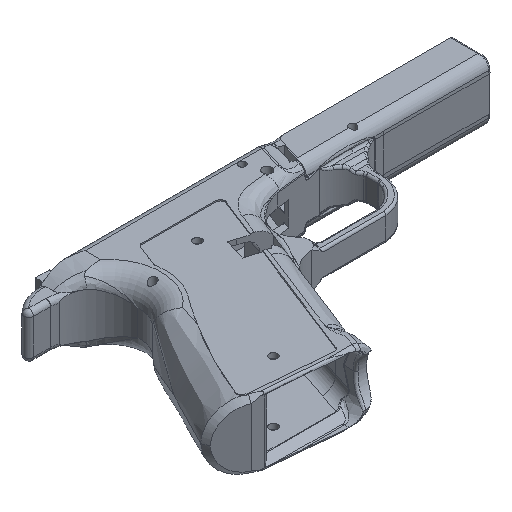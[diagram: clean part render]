
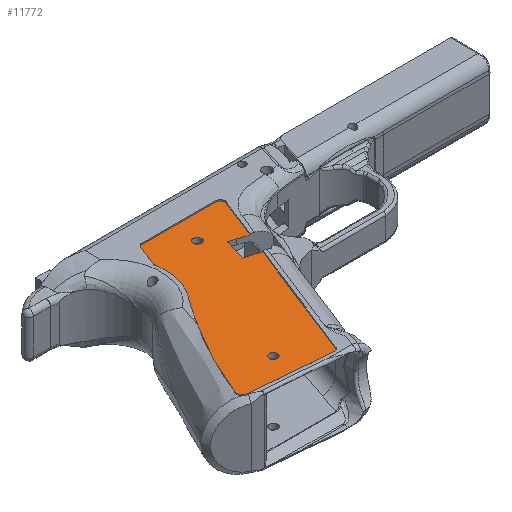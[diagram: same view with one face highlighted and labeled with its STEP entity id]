
A CAD part, isometric view. The second image highlights one B-rep face of the part: STEP entity #11772.
In plain terms, the highlighted planar face has unit normal (0, 0, 1).
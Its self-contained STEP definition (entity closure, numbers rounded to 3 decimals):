
#159=FACE_BOUND('',#2811,.T.);
#160=FACE_BOUND('',#2812,.T.);
#457=B_SPLINE_CURVE_WITH_KNOTS('',3,(#16690,#16691,#16692,#16693),
 .UNSPECIFIED.,.F.,.F.,(4,4),(1.719,2.121),
 .UNSPECIFIED.);
#1124=CIRCLE('',#11847,2.);
#1127=CIRCLE('',#11852,205.915);
#1274=CIRCLE('',#12141,2.);
#1275=CIRCLE('',#12143,22.827);
#1276=CIRCLE('',#12145,2.);
#1277=CIRCLE('',#12149,2.);
#1278=CIRCLE('',#12151,205.915);
#1279=CIRCLE('',#12153,2.);
#1280=CIRCLE('',#12156,2.);
#1281=CIRCLE('',#12162,21.378);
#1524=CIRCLE('',#12781,1.75);
#1526=CIRCLE('',#12784,1.75);
#2159=FACE_OUTER_BOUND('',#2810,.T.);
#2810=EDGE_LOOP('',(#10894,#10895,#10896,#10897,#10898,#10899,#10900,#10901,
#10902,#10903,#10904,#10905,#10906,#10907,#10908,#10909,#10910,#10911,#10912,
#10913));
#2811=EDGE_LOOP('',(#10914));
#2812=EDGE_LOOP('',(#10915));
#3101=LINE('',#24441,#3852);
#3103=LINE('',#24446,#3854);
#3109=LINE('',#24464,#3860);
#3111=LINE('',#24468,#3862);
#3115=LINE('',#24481,#3866);
#3116=LINE('',#24485,#3867);
#3117=LINE('',#24488,#3868);
#3226=LINE('',#29078,#3977);
#3246=LINE('',#29541,#3997);
#3852=VECTOR('',#13776,10.);
#3854=VECTOR('',#13780,10.);
#3860=VECTOR('',#13800,10.);
#3862=VECTOR('',#13804,10.);
#3866=VECTOR('',#13822,10.);
#3867=VECTOR('',#13829,10.);
#3868=VECTOR('',#13832,10.);
#3977=VECTOR('',#14211,10.);
#3997=VECTOR('',#14275,10.);
#4429=VERTEX_POINT('',#16684);
#4430=VERTEX_POINT('',#16689);
#4471=VERTEX_POINT('',#17024);
#4472=VERTEX_POINT('',#17026);
#4479=VERTEX_POINT('',#17115);
#4898=VERTEX_POINT('',#24437);
#4899=VERTEX_POINT('',#24439);
#4900=VERTEX_POINT('',#24443);
#4901=VERTEX_POINT('',#24445);
#4902=VERTEX_POINT('',#24449);
#4903=VERTEX_POINT('',#24450);
#4904=VERTEX_POINT('',#24457);
#4905=VERTEX_POINT('',#24458);
#4906=VERTEX_POINT('',#24463);
#4907=VERTEX_POINT('',#24467);
#4908=VERTEX_POINT('',#24471);
#4909=VERTEX_POINT('',#24477);
#4910=VERTEX_POINT('',#24487);
#4919=VERTEX_POINT('',#24523);
#5103=VERTEX_POINT('',#29077);
#5481=VERTEX_POINT('',#37650);
#5483=VERTEX_POINT('',#37656);
#5615=EDGE_CURVE('',#4429,#4430,#457,.T.);
#5663=EDGE_CURVE('',#4471,#4472,#1124,.T.);
#5672=EDGE_CURVE('',#4479,#4430,#1127,.T.);
#6277=EDGE_CURVE('',#4898,#4899,#3101,.T.);
#6279=EDGE_CURVE('',#4901,#4900,#3103,.T.);
#6281=EDGE_CURVE('',#4902,#4903,#1274,.T.);
#6284=EDGE_CURVE('',#4902,#4479,#1275,.T.);
#6285=EDGE_CURVE('',#4904,#4905,#1276,.T.);
#6288=EDGE_CURVE('',#4906,#4905,#3109,.T.);
#6290=EDGE_CURVE('',#4907,#4472,#3111,.T.);
#6292=EDGE_CURVE('',#4907,#4908,#1277,.T.);
#6294=EDGE_CURVE('',#4429,#4908,#1278,.T.);
#6295=EDGE_CURVE('',#4901,#4909,#1279,.T.);
#6297=EDGE_CURVE('',#4471,#4909,#3115,.T.);
#6298=EDGE_CURVE('',#4906,#4899,#1280,.T.);
#6299=EDGE_CURVE('',#4904,#4903,#3116,.T.);
#6300=EDGE_CURVE('',#4910,#4898,#3117,.T.);
#6310=EDGE_CURVE('',#4919,#4910,#1281,.T.);
#6587=EDGE_CURVE('',#5103,#4919,#3226,.T.);
#6622=EDGE_CURVE('',#4900,#5103,#3246,.T.);
#7296=EDGE_CURVE('',#5481,#5481,#1524,.T.);
#7299=EDGE_CURVE('',#5483,#5483,#1526,.T.);
#10894=ORIENTED_EDGE('',*,*,#5615,.F.);
#10895=ORIENTED_EDGE('',*,*,#6294,.T.);
#10896=ORIENTED_EDGE('',*,*,#6292,.F.);
#10897=ORIENTED_EDGE('',*,*,#6290,.T.);
#10898=ORIENTED_EDGE('',*,*,#5663,.F.);
#10899=ORIENTED_EDGE('',*,*,#6297,.T.);
#10900=ORIENTED_EDGE('',*,*,#6295,.F.);
#10901=ORIENTED_EDGE('',*,*,#6279,.T.);
#10902=ORIENTED_EDGE('',*,*,#6622,.T.);
#10903=ORIENTED_EDGE('',*,*,#6587,.T.);
#10904=ORIENTED_EDGE('',*,*,#6310,.T.);
#10905=ORIENTED_EDGE('',*,*,#6300,.T.);
#10906=ORIENTED_EDGE('',*,*,#6277,.T.);
#10907=ORIENTED_EDGE('',*,*,#6298,.F.);
#10908=ORIENTED_EDGE('',*,*,#6288,.T.);
#10909=ORIENTED_EDGE('',*,*,#6285,.F.);
#10910=ORIENTED_EDGE('',*,*,#6299,.T.);
#10911=ORIENTED_EDGE('',*,*,#6281,.F.);
#10912=ORIENTED_EDGE('',*,*,#6284,.T.);
#10913=ORIENTED_EDGE('',*,*,#5672,.T.);
#10914=ORIENTED_EDGE('',*,*,#7296,.F.);
#10915=ORIENTED_EDGE('',*,*,#7299,.F.);
#11138=PLANE('',#12785);
#11772=ADVANCED_FACE('',(#2159,#159,#160),#11138,.T.);
#11847=AXIS2_PLACEMENT_3D('',#17027,#12982,#12983);
#11852=AXIS2_PLACEMENT_3D('',#17116,#12993,#12994);
#12141=AXIS2_PLACEMENT_3D('',#24451,#13784,#13785);
#12143=AXIS2_PLACEMENT_3D('',#24455,#13790,#13791);
#12145=AXIS2_PLACEMENT_3D('',#24459,#13794,#13795);
#12149=AXIS2_PLACEMENT_3D('',#24472,#13808,#13809);
#12151=AXIS2_PLACEMENT_3D('',#24475,#13813,#13814);
#12153=AXIS2_PLACEMENT_3D('',#24478,#13817,#13818);
#12156=AXIS2_PLACEMENT_3D('',#24483,#13825,#13826);
#12162=AXIS2_PLACEMENT_3D('',#24524,#13844,#13845);
#12781=AXIS2_PLACEMENT_3D('',#37652,#15525,#15526);
#12784=AXIS2_PLACEMENT_3D('',#37658,#15532,#15533);
#12785=AXIS2_PLACEMENT_3D('',#37659,#15534,#15535);
#12982=DIRECTION('center_axis',(0.,0.,-1.));
#12983=DIRECTION('ref_axis',(-0.432,-0.902,0.));
#12993=DIRECTION('center_axis',(0.,0.,1.));
#12994=DIRECTION('ref_axis',(-0.93,0.367,0.));
#13776=DIRECTION('',(0.367,0.93,0.));
#13780=DIRECTION('',(0.367,0.93,0.));
#13784=DIRECTION('center_axis',(0.,0.,-1.));
#13785=DIRECTION('ref_axis',(-0.995,0.099,0.));
#13790=DIRECTION('center_axis',(0.,0.,-1.));
#13791=DIRECTION('ref_axis',(0.98,0.2,0.));
#13794=DIRECTION('center_axis',(0.,0.,-1.));
#13795=DIRECTION('ref_axis',(-0.563,0.827,0.));
#13800=DIRECTION('',(-1.,0.,0.));
#13804=DIRECTION('',(0.694,-0.72,0.));
#13808=DIRECTION('center_axis',(0.,0.,-1.));
#13809=DIRECTION('ref_axis',(-0.982,-0.191,0.));
#13813=DIRECTION('center_axis',(0.,0.,1.));
#13814=DIRECTION('ref_axis',(-0.93,0.367,0.));
#13817=DIRECTION('center_axis',(0.,0.,-1.));
#13818=DIRECTION('ref_axis',(0.525,-0.851,0.));
#13822=DIRECTION('',(0.996,-0.089,0.));
#13825=DIRECTION('center_axis',(0.,0.,-1.));
#13826=DIRECTION('ref_axis',(0.827,0.563,0.));
#13829=DIRECTION('',(-0.367,-0.93,0.));
#13832=DIRECTION('',(0.954,-0.301,0.));
#13844=DIRECTION('center_axis',(0.,0.,-1.));
#13845=DIRECTION('ref_axis',(0.383,0.924,0.));
#14211=DIRECTION('',(0.301,0.954,0.));
#14275=DIRECTION('',(-0.954,0.301,0.));
#15525=DIRECTION('center_axis',(0.,0.,1.));
#15526=DIRECTION('ref_axis',(-1.,0.,0.));
#15532=DIRECTION('center_axis',(0.,0.,1.));
#15533=DIRECTION('ref_axis',(-1.,0.,0.));
#15534=DIRECTION('center_axis',(0.,0.,1.));
#15535=DIRECTION('ref_axis',(-1.,0.,0.));
#16684=CARTESIAN_POINT('',(2.289,-72.023,13.9));
#16689=CARTESIAN_POINT('',(3.33,-69.939,13.9));
#16690=CARTESIAN_POINT('Ctrl Pts',(2.289,-72.023,13.9));
#16691=CARTESIAN_POINT('Ctrl Pts',(2.675,-71.28,13.9));
#16692=CARTESIAN_POINT('Ctrl Pts',(3.013,-70.609,13.9));
#16693=CARTESIAN_POINT('Ctrl Pts',(3.33,-69.939,13.9));
#17024=CARTESIAN_POINT('',(-1.911,-89.531,13.9));
#17026=CARTESIAN_POINT('',(-3.174,-88.926,13.9));
#17027=CARTESIAN_POINT('Origin',(-1.733,-87.539,13.9));
#17115=CARTESIAN_POINT('',(20.96,-41.234,13.9));
#17116=CARTESIAN_POINT('Origin',(187.022,-162.989,13.9));
#24437=CARTESIAN_POINT('',(56.284,-32.004,13.9));
#24439=CARTESIAN_POINT('',(62.767,-15.546,13.9));
#24441=CARTESIAN_POINT('',(63.843,-12.813,13.9));
#24443=CARTESIAN_POINT('',(52.831,-40.771,13.9));
#24445=CARTESIAN_POINT('',(32.964,-91.204,13.9));
#24446=CARTESIAN_POINT('',(63.843,-12.813,13.9));
#24449=CARTESIAN_POINT('',(24.96,-23.806,13.9));
#24450=CARTESIAN_POINT('',(25.068,-22.722,13.9));
#24451=CARTESIAN_POINT('Origin',(26.929,-23.455,13.9));
#24455=CARTESIAN_POINT('Origin',(2.489,-27.821,13.9));
#24457=CARTESIAN_POINT('',(28.472,-14.08,13.9));
#24458=CARTESIAN_POINT('',(30.333,-12.813,13.9));
#24459=CARTESIAN_POINT('Origin',(30.333,-14.813,13.9));
#24463=CARTESIAN_POINT('',(60.906,-12.813,13.9));
#24464=CARTESIAN_POINT('',(28.971,-12.813,13.9));
#24467=CARTESIAN_POINT('',(-3.66,-88.422,13.9));
#24468=CARTESIAN_POINT('',(-2.655,-89.464,13.9));
#24471=CARTESIAN_POINT('',(-4.076,-86.289,13.9));
#24472=CARTESIAN_POINT('Origin',(-2.22,-87.034,13.9));
#24475=CARTESIAN_POINT('Origin',(187.022,-162.989,13.9));
#24477=CARTESIAN_POINT('',(30.926,-92.463,13.9));
#24478=CARTESIAN_POINT('Origin',(31.104,-90.471,13.9));
#24481=CARTESIAN_POINT('',(32.416,-92.596,13.9));
#24483=CARTESIAN_POINT('Origin',(60.906,-14.813,13.9));
#24485=CARTESIAN_POINT('',(24.856,-23.261,13.9));
#24487=CARTESIAN_POINT('',(52.066,-30.673,13.9));
#24488=CARTESIAN_POINT('',(51.56,-30.514,13.9));
#24523=CARTESIAN_POINT('',(49.097,-29.689,13.9));
#24524=CARTESIAN_POINT('Origin',(43.871,-50.418,13.9));
#29077=CARTESIAN_POINT('',(46.257,-38.698,13.9));
#29078=CARTESIAN_POINT('',(47.47,-34.852,13.9));
#29541=CARTESIAN_POINT('',(43.774,-37.915,13.9));
#37650=CARTESIAN_POINT('',(44.882,-23.118,13.9));
#37652=CARTESIAN_POINT('Origin',(43.132,-23.118,13.9));
#37656=CARTESIAN_POINT('',(19.042,-80.791,13.9));
#37658=CARTESIAN_POINT('Origin',(17.292,-80.791,13.9));
#37659=CARTESIAN_POINT('Origin',(29.343,-52.642,13.9));
